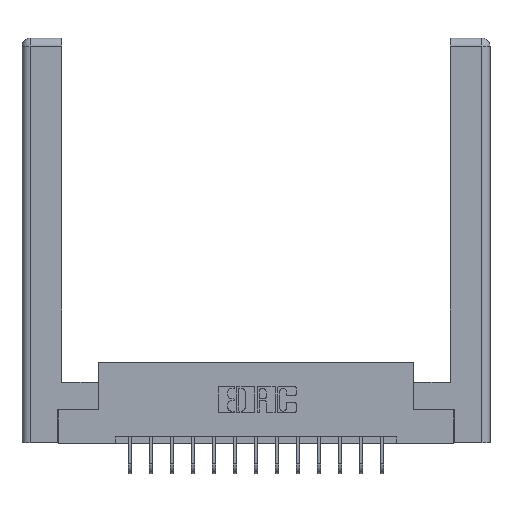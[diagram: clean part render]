
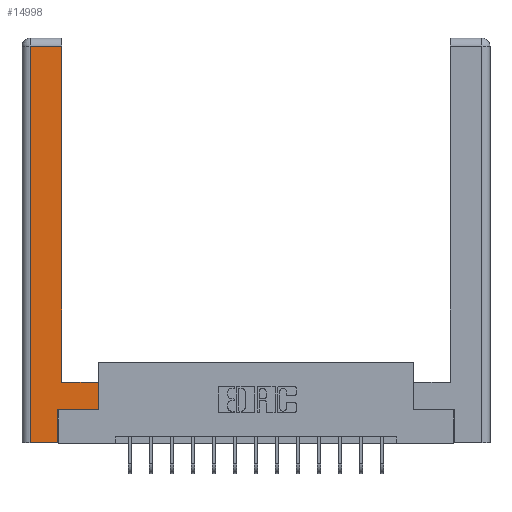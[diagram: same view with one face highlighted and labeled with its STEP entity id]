
A CAD part, top view. The second image highlights one B-rep face of the part: STEP entity #14998.
In plain terms, the highlighted planar face has unit normal (0, 0, 1).
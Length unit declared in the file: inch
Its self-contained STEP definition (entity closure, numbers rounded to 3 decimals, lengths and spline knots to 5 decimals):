
#183 = VERTEX_POINT ( 'NONE', #10643 ) ;
#869 = VECTOR ( 'NONE', #3411, 39.37008 ) ;
#1259 = ORIENTED_EDGE ( 'NONE', *, *, #4792, .T. ) ;
#1470 = VERTEX_POINT ( 'NONE', #10942 ) ;
#1519 = LINE ( 'NONE', #14546, #11468 ) ;
#1900 = VECTOR ( 'NONE', #5846, 39.37008 ) ;
#2043 = ORIENTED_EDGE ( 'NONE', *, *, #12696, .T. ) ;
#2142 = CARTESIAN_POINT ( 'NONE',  ( 0., 0., 0. ) ) ;
#2171 = LINE ( 'NONE', #11415, #9254 ) ;
#2960 = DIRECTION ( 'NONE',  ( 0., 1., 0. ) ) ;
#2969 = FACE_OUTER_BOUND ( 'NONE', #16628, .T. ) ;
#3090 = CARTESIAN_POINT ( 'NONE',  ( 0.295, 3., 0. ) ) ;
#3124 = CARTESIAN_POINT ( 'NONE',  ( 0.265, 0., 0. ) ) ;
#3282 = DIRECTION ( 'NONE',  ( -1., 0., 0. ) ) ;
#3411 = DIRECTION ( 'NONE',  ( 0., -1., 0. ) ) ;
#3453 = CARTESIAN_POINT ( 'NONE',  ( 0.265, 0., 0. ) ) ;
#3916 = DIRECTION ( 'NONE',  ( 0., 0., -1. ) ) ;
#4408 = DIRECTION ( 'NONE',  ( 0., 1., 0. ) ) ;
#4516 = VECTOR ( 'NONE', #3282, 39.37008 ) ;
#4792 = EDGE_CURVE ( 'NONE', #16403, #6134, #2171, .T. ) ;
#4815 = LINE ( 'NONE', #3124, #15587 ) ;
#4862 = AXIS2_PLACEMENT_3D ( 'NONE', #2142, #3916, #10909 ) ;
#5705 = EDGE_CURVE ( 'NONE', #14216, #16403, #4815, .T. ) ;
#5846 = DIRECTION ( 'NONE',  ( 0., 1., 0. ) ) ;
#6134 = VERTEX_POINT ( 'NONE', #6198 ) ;
#6198 = CARTESIAN_POINT ( 'NONE',  ( 0.265, 0.245, 0. ) ) ;
#6492 = LINE ( 'NONE', #15962, #4516 ) ;
#6692 = ORIENTED_EDGE ( 'NONE', *, *, #5705, .T. ) ;
#7137 = DIRECTION ( 'NONE',  ( 1., 0., 0. ) ) ;
#7206 = ORIENTED_EDGE ( 'NONE', *, *, #14689, .T. ) ;
#7366 = VERTEX_POINT ( 'NONE', #11376 ) ;
#7467 = DIRECTION ( 'NONE',  ( 1., 0., 0. ) ) ;
#8063 = ORIENTED_EDGE ( 'NONE', *, *, #17533, .T. ) ;
#8412 = LINE ( 'NONE', #12218, #11260 ) ;
#9254 = VECTOR ( 'NONE', #2960, 39.37008 ) ;
#9392 = DIRECTION ( 'NONE',  ( -1., 0., 0. ) ) ;
#9529 = CARTESIAN_POINT ( 'NONE',  ( 0.0615, 0., 0. ) ) ;
#9708 = PLANE ( 'NONE',  #4862 ) ;
#10643 = CARTESIAN_POINT ( 'NONE',  ( 0.295, 2.94, 0. ) ) ;
#10723 = ORIENTED_EDGE ( 'NONE', *, *, #12039, .T. ) ;
#10909 = DIRECTION ( 'NONE',  ( -1., 0., 0. ) ) ;
#10942 = CARTESIAN_POINT ( 'NONE',  ( 0.565, 0.45, 0. ) ) ;
#10954 = VERTEX_POINT ( 'NONE', #11051 ) ;
#11051 = CARTESIAN_POINT ( 'NONE',  ( 0.0615, 2.94, 0. ) ) ;
#11260 = VECTOR ( 'NONE', #9392, 39.37008 ) ;
#11376 = CARTESIAN_POINT ( 'NONE',  ( 0.565, 0.245, 0. ) ) ;
#11409 = VERTEX_POINT ( 'NONE', #13371 ) ;
#11415 = CARTESIAN_POINT ( 'NONE',  ( 0.265, 0.245, 0. ) ) ;
#11468 = VECTOR ( 'NONE', #7467, 39.37008 ) ;
#12039 = EDGE_CURVE ( 'NONE', #6134, #7366, #1519, .T. ) ;
#12069 = ORIENTED_EDGE ( 'NONE', *, *, #13457, .T. ) ;
#12218 = CARTESIAN_POINT ( 'NONE',  ( 0.0615, 2.94, 0. ) ) ;
#12696 = EDGE_CURVE ( 'NONE', #11409, #183, #15161, .T. ) ;
#12984 = VECTOR ( 'NONE', #4408, 39.37008 ) ;
#13222 = CARTESIAN_POINT ( 'NONE',  ( 0.0615, 0., 0. ) ) ;
#13371 = CARTESIAN_POINT ( 'NONE',  ( 0.295, 0.45, 0. ) ) ;
#13391 = LINE ( 'NONE', #15498, #1900 ) ;
#13457 = EDGE_CURVE ( 'NONE', #7366, #1470, #13391, .T. ) ;
#14216 = VERTEX_POINT ( 'NONE', #9529 ) ;
#14546 = CARTESIAN_POINT ( 'NONE',  ( 0.565, 0.245, 0. ) ) ;
#14553 = LINE ( 'NONE', #13222, #869 ) ;
#14689 = EDGE_CURVE ( 'NONE', #1470, #11409, #6492, .T. ) ;
#14998 = ADVANCED_FACE ( 'NONE', ( #2969 ), #9708, .F. ) ;
#15161 = LINE ( 'NONE', #3090, #12984 ) ;
#15498 = CARTESIAN_POINT ( 'NONE',  ( 0.565, 0.45, 0. ) ) ;
#15587 = VECTOR ( 'NONE', #7137, 39.37008 ) ;
#15962 = CARTESIAN_POINT ( 'NONE',  ( 0.295, 0.45, 0. ) ) ;
#16403 = VERTEX_POINT ( 'NONE', #3453 ) ;
#16628 = EDGE_LOOP ( 'NONE', ( #2043, #17721, #8063, #6692, #1259, #10723, #12069, #7206 ) ) ;
#17533 = EDGE_CURVE ( 'NONE', #10954, #14216, #14553, .T. ) ;
#17603 = EDGE_CURVE ( 'NONE', #183, #10954, #8412, .T. ) ;
#17721 = ORIENTED_EDGE ( 'NONE', *, *, #17603, .T. ) ;
